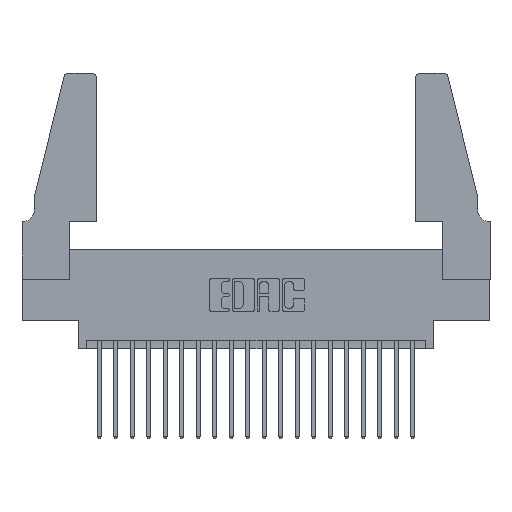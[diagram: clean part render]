
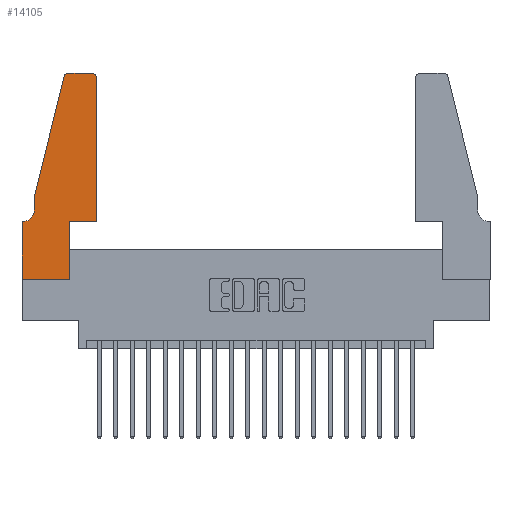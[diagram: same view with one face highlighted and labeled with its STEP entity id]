
A CAD part, top view. The second image highlights one B-rep face of the part: STEP entity #14105.
In plain terms, the highlighted planar face has unit normal (0, 0, 1).
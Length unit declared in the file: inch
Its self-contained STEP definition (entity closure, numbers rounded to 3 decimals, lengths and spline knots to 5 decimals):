
#78 = ORIENTED_EDGE ( 'NONE', *, *, #20658, .T. ) ;
#334 = CARTESIAN_POINT ( 'NONE',  ( 0., 0., 0.37 ) ) ;
#613 = ORIENTED_EDGE ( 'NONE', *, *, #8223, .T. ) ;
#738 = CARTESIAN_POINT ( 'NONE',  ( 0.284, 1.22, 0.37 ) ) ;
#752 = CARTESIAN_POINT ( 'NONE',  ( 0., 0., 0.37 ) ) ;
#762 = CARTESIAN_POINT ( 'NONE',  ( 0., 0.35, 0.37 ) ) ;
#850 = DIRECTION ( 'NONE',  ( 1., 0., 0. ) ) ;
#999 = LINE ( 'NONE', #1596, #20962 ) ;
#1187 = EDGE_CURVE ( 'NONE', #4353, #2596, #2668, .T. ) ;
#1232 = DIRECTION ( 'NONE',  ( 1., 0., 0. ) ) ;
#1237 = LINE ( 'NONE', #15084, #18215 ) ;
#1473 = AXIS2_PLACEMENT_3D ( 'NONE', #20835, #11298, #1516 ) ;
#1516 = DIRECTION ( 'NONE',  ( -1., 0., 0. ) ) ;
#1596 = CARTESIAN_POINT ( 'NONE',  ( 0.2865, 0.35, 0.37 ) ) ;
#1767 = CARTESIAN_POINT ( 'NONE',  ( 0.2865, 0., 0.37 ) ) ;
#2249 = ORIENTED_EDGE ( 'NONE', *, *, #13887, .T. ) ;
#2346 = DIRECTION ( 'NONE',  ( -0.239, -0.971, 0. ) ) ;
#2495 = DIRECTION ( 'NONE',  ( 1., 0., 0. ) ) ;
#2596 = VERTEX_POINT ( 'NONE', #334 ) ;
#2639 = CARTESIAN_POINT ( 'NONE',  ( 0., 0., 0.37 ) ) ;
#2668 = LINE ( 'NONE', #2639, #10778 ) ;
#2948 = VERTEX_POINT ( 'NONE', #5111 ) ;
#3571 = VERTEX_POINT ( 'NONE', #1767 ) ;
#3690 = LINE ( 'NONE', #8726, #19169 ) ;
#4183 = VERTEX_POINT ( 'NONE', #4847 ) ;
#4353 = VERTEX_POINT ( 'NONE', #14873 ) ;
#4469 = VERTEX_POINT ( 'NONE', #19991 ) ;
#4488 = EDGE_CURVE ( 'NONE', #10990, #4183, #16411, .T. ) ;
#4847 = CARTESIAN_POINT ( 'NONE',  ( 0.0755, 0.5, 0.37 ) ) ;
#4935 = DIRECTION ( 'NONE',  ( 0., -1., 0. ) ) ;
#5111 = CARTESIAN_POINT ( 'NONE',  ( 0.0055, 0.35, 0.37 ) ) ;
#5126 = ORIENTED_EDGE ( 'NONE', *, *, #8473, .T. ) ;
#5225 = AXIS2_PLACEMENT_3D ( 'NONE', #762, #5871, #17010 ) ;
#5550 = DIRECTION ( 'NONE',  ( 0., 1., 0. ) ) ;
#5871 = DIRECTION ( 'NONE',  ( 0., 0., 1. ) ) ;
#6418 = EDGE_CURVE ( 'NONE', #10074, #10990, #8858, .T. ) ;
#7331 = AXIS2_PLACEMENT_3D ( 'NONE', #738, #12191, #2495 ) ;
#8059 = VERTEX_POINT ( 'NONE', #10881 ) ;
#8100 = EDGE_LOOP ( 'NONE', ( #12137, #16397, #16883, #78, #613, #5126, #9881, #14144, #2249, #15658, #19867, #11901 ) ) ;
#8223 = EDGE_CURVE ( 'NONE', #16711, #2948, #11231, .T. ) ;
#8473 = EDGE_CURVE ( 'NONE', #2948, #4353, #1237, .T. ) ;
#8560 = EDGE_CURVE ( 'NONE', #4469, #10074, #17229, .T. ) ;
#8726 = CARTESIAN_POINT ( 'NONE',  ( 0.4505, 0.35, 0.37 ) ) ;
#8858 = CIRCLE ( 'NONE', #7331, 0.03 ) ;
#9330 = AXIS2_PLACEMENT_3D ( 'NONE', #20573, #11037, #1232 ) ;
#9792 = LINE ( 'NONE', #752, #18268 ) ;
#9881 = ORIENTED_EDGE ( 'NONE', *, *, #1187, .T. ) ;
#9927 = EDGE_CURVE ( 'NONE', #20730, #4469, #14192, .T. ) ;
#10074 = VERTEX_POINT ( 'NONE', #14605 ) ;
#10520 = CARTESIAN_POINT ( 'NONE',  ( 0.2605, 1.25, 0.37 ) ) ;
#10778 = VECTOR ( 'NONE', #17293, 39.37008 ) ;
#10881 = CARTESIAN_POINT ( 'NONE',  ( 0.4505, 0.35, 0.37 ) ) ;
#10938 = VERTEX_POINT ( 'NONE', #18093 ) ;
#10990 = VERTEX_POINT ( 'NONE', #16665 ) ;
#11037 = DIRECTION ( 'NONE',  ( 0., 0., 1. ) ) ;
#11231 = CIRCLE ( 'NONE', #1473, 0.07 ) ;
#11298 = DIRECTION ( 'NONE',  ( 0., 0., -1. ) ) ;
#11439 = CARTESIAN_POINT ( 'NONE',  ( 0.0755, 0.42, 0.37 ) ) ;
#11657 = VECTOR ( 'NONE', #2346, 39.37008 ) ;
#11901 = ORIENTED_EDGE ( 'NONE', *, *, #9927, .T. ) ;
#12137 = ORIENTED_EDGE ( 'NONE', *, *, #8560, .T. ) ;
#12191 = DIRECTION ( 'NONE',  ( 0., 0., 1. ) ) ;
#12202 = DIRECTION ( 'NONE',  ( 1., 0., 0. ) ) ;
#12293 = CARTESIAN_POINT ( 'NONE',  ( 0.4505, 0.35, 0.37 ) ) ;
#12660 = VECTOR ( 'NONE', #4935, 39.37008 ) ;
#12737 = FACE_OUTER_BOUND ( 'NONE', #8100, .T. ) ;
#13046 = VECTOR ( 'NONE', #850, 39.37008 ) ;
#13174 = LINE ( 'NONE', #16136, #12660 ) ;
#13831 = PLANE ( 'NONE',  #5225 ) ;
#13887 = EDGE_CURVE ( 'NONE', #3571, #10938, #999, .T. ) ;
#14105 = ADVANCED_FACE ( 'NONE', ( #12737 ), #13831, .T. ) ;
#14144 = ORIENTED_EDGE ( 'NONE', *, *, #19083, .T. ) ;
#14192 = CIRCLE ( 'NONE', #9330, 0.03 ) ;
#14605 = CARTESIAN_POINT ( 'NONE',  ( 0.284, 1.25, 0.37 ) ) ;
#14609 = EDGE_CURVE ( 'NONE', #8059, #20730, #3690, .T. ) ;
#14676 = CARTESIAN_POINT ( 'NONE',  ( 0.4505, 1.22, 0.37 ) ) ;
#14873 = CARTESIAN_POINT ( 'NONE',  ( 0., 0.35, 0.37 ) ) ;
#15084 = CARTESIAN_POINT ( 'NONE',  ( 0.0755, 0.35, 0.37 ) ) ;
#15219 = CARTESIAN_POINT ( 'NONE',  ( 0.0755, 0.5, 0.37 ) ) ;
#15658 = ORIENTED_EDGE ( 'NONE', *, *, #18510, .T. ) ;
#16136 = CARTESIAN_POINT ( 'NONE',  ( 0.0755, 0.5, 0.37 ) ) ;
#16294 = LINE ( 'NONE', #12293, #13046 ) ;
#16397 = ORIENTED_EDGE ( 'NONE', *, *, #6418, .T. ) ;
#16411 = LINE ( 'NONE', #15219, #11657 ) ;
#16665 = CARTESIAN_POINT ( 'NONE',  ( 0.25487, 1.22718, 0.37 ) ) ;
#16711 = VERTEX_POINT ( 'NONE', #11439 ) ;
#16883 = ORIENTED_EDGE ( 'NONE', *, *, #4488, .T. ) ;
#17010 = DIRECTION ( 'NONE',  ( 1., 0., 0. ) ) ;
#17229 = LINE ( 'NONE', #10520, #20958 ) ;
#17293 = DIRECTION ( 'NONE',  ( 0., -1., 0. ) ) ;
#17776 = DIRECTION ( 'NONE',  ( 0., 1., 0. ) ) ;
#18093 = CARTESIAN_POINT ( 'NONE',  ( 0.2865, 0.35, 0.37 ) ) ;
#18215 = VECTOR ( 'NONE', #18242, 39.37008 ) ;
#18242 = DIRECTION ( 'NONE',  ( -1., 0., 0. ) ) ;
#18268 = VECTOR ( 'NONE', #12202, 39.37008 ) ;
#18510 = EDGE_CURVE ( 'NONE', #10938, #8059, #16294, .T. ) ;
#19083 = EDGE_CURVE ( 'NONE', #2596, #3571, #9792, .T. ) ;
#19169 = VECTOR ( 'NONE', #5550, 39.37008 ) ;
#19867 = ORIENTED_EDGE ( 'NONE', *, *, #14609, .T. ) ;
#19991 = CARTESIAN_POINT ( 'NONE',  ( 0.4205, 1.25, 0.37 ) ) ;
#20066 = DIRECTION ( 'NONE',  ( -1., 0., 0. ) ) ;
#20573 = CARTESIAN_POINT ( 'NONE',  ( 0.4205, 1.22, 0.37 ) ) ;
#20658 = EDGE_CURVE ( 'NONE', #4183, #16711, #13174, .T. ) ;
#20730 = VERTEX_POINT ( 'NONE', #14676 ) ;
#20835 = CARTESIAN_POINT ( 'NONE',  ( 0.0055, 0.42, 0.37 ) ) ;
#20958 = VECTOR ( 'NONE', #20066, 39.37008 ) ;
#20962 = VECTOR ( 'NONE', #17776, 39.37008 ) ;
